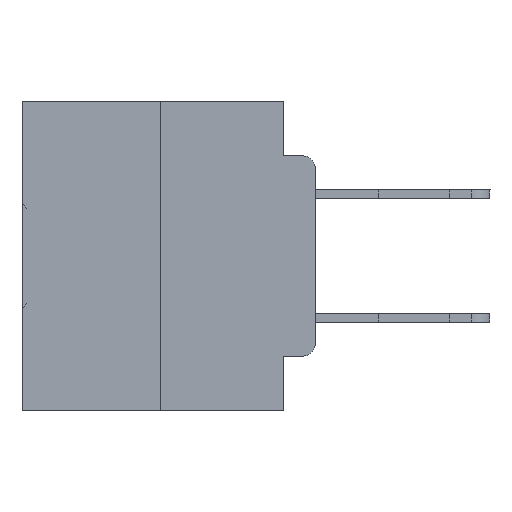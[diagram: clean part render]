
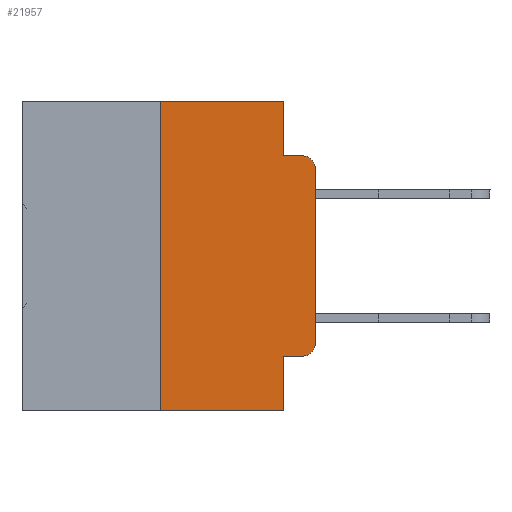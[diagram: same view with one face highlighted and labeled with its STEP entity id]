
A CAD part, left-side view. The second image highlights one B-rep face of the part: STEP entity #21957.
In plain terms, the highlighted planar face has unit normal (-1, 0, 0).
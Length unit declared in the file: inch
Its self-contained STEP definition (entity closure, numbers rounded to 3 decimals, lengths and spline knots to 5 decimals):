
#105 = CARTESIAN_POINT ( 'NONE',  ( 0., 0.473, 0. ) ) ;
#315 = DIRECTION ( 'NONE',  ( 0., -1., 0. ) ) ;
#702 = LINE ( 'NONE', #23109, #5857 ) ;
#1116 = VERTEX_POINT ( 'NONE', #23427 ) ;
#2355 = DIRECTION ( 'NONE',  ( 0., -1., 0. ) ) ;
#2575 = VERTEX_POINT ( 'NONE', #11880 ) ;
#5315 = LINE ( 'NONE', #5662, #32161 ) ;
#5662 = CARTESIAN_POINT ( 'NONE',  ( 0., 0.25, 0. ) ) ;
#5857 = VECTOR ( 'NONE', #8973, 39.37008 ) ;
#6215 = CARTESIAN_POINT ( 'NONE',  ( 0., 0., -0.3915 ) ) ;
#7922 = CARTESIAN_POINT ( 'NONE',  ( 0., 0., -0.1085 ) ) ;
#8155 = DIRECTION ( 'NONE',  ( 0., 0., 1. ) ) ;
#8329 = CARTESIAN_POINT ( 'NONE',  ( 0., 0.051, -0.5 ) ) ;
#8973 = DIRECTION ( 'NONE',  ( 0., 0., -1. ) ) ;
#9655 = DIRECTION ( 'NONE',  ( 0., -1., 0. ) ) ;
#10520 = CARTESIAN_POINT ( 'NONE',  ( 0., 0., 0. ) ) ;
#10952 = AXIS2_PLACEMENT_3D ( 'NONE', #30450, #19874, #16840 ) ;
#11656 = LINE ( 'NONE', #13981, #22959 ) ;
#11880 = CARTESIAN_POINT ( 'NONE',  ( 0., 0.051, -0.4115 ) ) ;
#11926 = VERTEX_POINT ( 'NONE', #19484 ) ;
#12144 = VECTOR ( 'NONE', #15282, 39.37008 ) ;
#12253 = VECTOR ( 'NONE', #25700, 39.37008 ) ;
#12514 = ORIENTED_EDGE ( 'NONE', *, *, #23734, .F. ) ;
#12671 = CIRCLE ( 'NONE', #10952, 0.02 ) ;
#12718 = VECTOR ( 'NONE', #8155, 39.37008 ) ;
#12780 = CARTESIAN_POINT ( 'NONE',  ( 0., 0.051, -0.4115 ) ) ;
#13460 = EDGE_CURVE ( 'NONE', #11926, #34631, #12671, .T. ) ;
#13477 = EDGE_CURVE ( 'NONE', #32305, #16565, #11656, .T. ) ;
#13586 = DIRECTION ( 'NONE',  ( 1., 0., 0. ) ) ;
#13754 = FACE_OUTER_BOUND ( 'NONE', #14706, .T. ) ;
#13981 = CARTESIAN_POINT ( 'NONE',  ( 0., 0.051, -0.0885 ) ) ;
#14146 = EDGE_CURVE ( 'NONE', #34631, #28345, #32191, .T. ) ;
#14498 = ORIENTED_EDGE ( 'NONE', *, *, #23516, .T. ) ;
#14543 = CARTESIAN_POINT ( 'NONE',  ( 0., 0.051, 0. ) ) ;
#14595 = DIRECTION ( 'NONE',  ( 0., 0., -1. ) ) ;
#14706 = EDGE_LOOP ( 'NONE', ( #22858, #29485, #33464, #23406, #27918, #27542, #15587, #12514, #14498, #15763 ) ) ;
#15282 = DIRECTION ( 'NONE',  ( 0., -1., 0. ) ) ;
#15370 = VERTEX_POINT ( 'NONE', #14543 ) ;
#15587 = ORIENTED_EDGE ( 'NONE', *, *, #29511, .T. ) ;
#15763 = ORIENTED_EDGE ( 'NONE', *, *, #13460, .T. ) ;
#15814 = LINE ( 'NONE', #12780, #12144 ) ;
#15851 = VECTOR ( 'NONE', #2355, 39.37008 ) ;
#16141 = EDGE_CURVE ( 'NONE', #24550, #1116, #5315, .T. ) ;
#16273 = DIRECTION ( 'NONE',  ( 0., 0., 1. ) ) ;
#16565 = VERTEX_POINT ( 'NONE', #29468 ) ;
#16597 = EDGE_CURVE ( 'NONE', #28345, #16565, #33911, .T. ) ;
#16840 = DIRECTION ( 'NONE',  ( 0., 0., -1. ) ) ;
#17769 = VERTEX_POINT ( 'NONE', #8329 ) ;
#18446 = AXIS2_PLACEMENT_3D ( 'NONE', #19259, #27990, #14595 ) ;
#18524 = LINE ( 'NONE', #29605, #15851 ) ;
#18602 = CARTESIAN_POINT ( 'NONE',  ( 0., 0.25, -0.5 ) ) ;
#18871 = CARTESIAN_POINT ( 'NONE',  ( 0., 0.051, -0.0885 ) ) ;
#19030 = EDGE_CURVE ( 'NONE', #1116, #15370, #23251, .T. ) ;
#19259 = CARTESIAN_POINT ( 'NONE',  ( 0., 0.02, -0.1085 ) ) ;
#19484 = CARTESIAN_POINT ( 'NONE',  ( 0., 0.02, -0.4115 ) ) ;
#19874 = DIRECTION ( 'NONE',  ( -1., 0., 0. ) ) ;
#21957 = ADVANCED_FACE ( 'NONE', ( #13754 ), #29878, .F. ) ;
#22858 = ORIENTED_EDGE ( 'NONE', *, *, #14146, .T. ) ;
#22959 = VECTOR ( 'NONE', #315, 39.37008 ) ;
#23020 = AXIS2_PLACEMENT_3D ( 'NONE', #105, #13586, #23958 ) ;
#23023 = LINE ( 'NONE', #26236, #12253 ) ;
#23109 = CARTESIAN_POINT ( 'NONE',  ( 0., 0.051, 0. ) ) ;
#23251 = LINE ( 'NONE', #34219, #30540 ) ;
#23406 = ORIENTED_EDGE ( 'NONE', *, *, #24856, .F. ) ;
#23427 = CARTESIAN_POINT ( 'NONE',  ( 0., 0.25, 0. ) ) ;
#23516 = EDGE_CURVE ( 'NONE', #2575, #11926, #15814, .T. ) ;
#23734 = EDGE_CURVE ( 'NONE', #2575, #17769, #702, .T. ) ;
#23958 = DIRECTION ( 'NONE',  ( 0., 0., -1. ) ) ;
#24550 = VERTEX_POINT ( 'NONE', #18602 ) ;
#24856 = EDGE_CURVE ( 'NONE', #15370, #32305, #23023, .T. ) ;
#25700 = DIRECTION ( 'NONE',  ( 0., 0., -1. ) ) ;
#26236 = CARTESIAN_POINT ( 'NONE',  ( 0., 0.051, 0. ) ) ;
#27542 = ORIENTED_EDGE ( 'NONE', *, *, #16141, .F. ) ;
#27918 = ORIENTED_EDGE ( 'NONE', *, *, #19030, .F. ) ;
#27990 = DIRECTION ( 'NONE',  ( -1., 0., 0. ) ) ;
#28345 = VERTEX_POINT ( 'NONE', #7922 ) ;
#29468 = CARTESIAN_POINT ( 'NONE',  ( 0., 0.02, -0.0885 ) ) ;
#29485 = ORIENTED_EDGE ( 'NONE', *, *, #16597, .T. ) ;
#29511 = EDGE_CURVE ( 'NONE', #24550, #17769, #18524, .T. ) ;
#29605 = CARTESIAN_POINT ( 'NONE',  ( 0., 0.473, -0.5 ) ) ;
#29878 = PLANE ( 'NONE',  #23020 ) ;
#30450 = CARTESIAN_POINT ( 'NONE',  ( 0., 0.02, -0.3915 ) ) ;
#30540 = VECTOR ( 'NONE', #9655, 39.37008 ) ;
#32161 = VECTOR ( 'NONE', #16273, 39.37008 ) ;
#32191 = LINE ( 'NONE', #10520, #12718 ) ;
#32305 = VERTEX_POINT ( 'NONE', #18871 ) ;
#33464 = ORIENTED_EDGE ( 'NONE', *, *, #13477, .F. ) ;
#33911 = CIRCLE ( 'NONE', #18446, 0.02 ) ;
#34219 = CARTESIAN_POINT ( 'NONE',  ( 0., 0.473, 0. ) ) ;
#34631 = VERTEX_POINT ( 'NONE', #6215 ) ;
